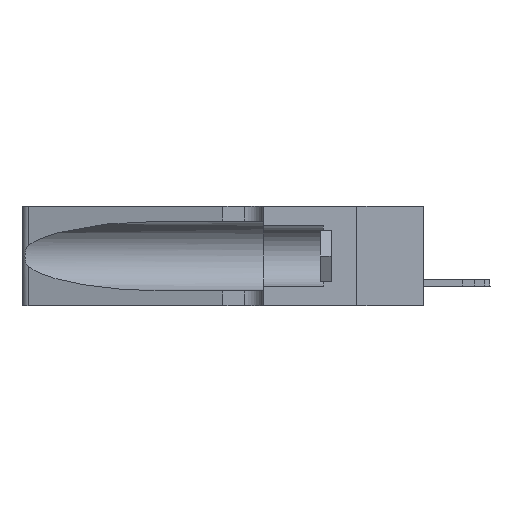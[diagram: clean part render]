
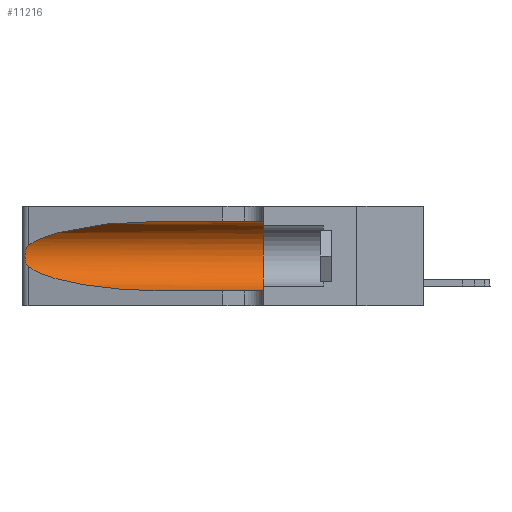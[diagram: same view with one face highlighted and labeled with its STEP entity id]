
A CAD part, left-side view. The second image highlights one B-rep face of the part: STEP entity #11216.
In plain terms, the highlighted cylindrical face has radius 3.308 mm (diameter 6.617 mm), a partial arc.
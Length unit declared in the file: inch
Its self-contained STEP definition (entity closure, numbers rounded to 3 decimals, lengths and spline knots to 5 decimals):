
#1610 = CYLINDRICAL_SURFACE ( 'NONE', #5016, 0.13025 ) ;
#2226 = DIRECTION ( 'NONE',  ( 0., 1., 0. ) ) ;
#2323 = DIRECTION ( 'NONE',  ( 0., 0., 1. ) ) ;
#2825 = AXIS2_PLACEMENT_3D ( 'NONE', #12289, #2226, #2323 ) ;
#3689 = ORIENTED_EDGE ( 'NONE', *, *, #10158, .T. ) ;
#3741 = ORIENTED_EDGE ( 'NONE', *, *, #10546, .T. ) ;
#3922 = CARTESIAN_POINT ( 'NONE',  ( 0.2373, 1.15595, 0.28018 ) ) ;
#4613 = CARTESIAN_POINT ( 'NONE',  ( 0.25787, 1.23484, 0.2124 ) ) ;
#5016 = AXIS2_PLACEMENT_3D ( 'NONE', #22524, #19921, #25355 ) ;
#5555 = CARTESIAN_POINT ( 'NONE',  ( 0.25487, 1.22718, 0.14631 ) ) ;
#5918 = EDGE_LOOP ( 'NONE', ( #3689, #3741, #30185, #19300, #8326, #10552 ) ) ;
#6093 = CARTESIAN_POINT ( 'NONE',  ( 0.1305, 0.72297, 0.31525 ) ) ;
#6492 = FACE_OUTER_BOUND ( 'NONE', #5918, .T. ) ;
#6548 = CARTESIAN_POINT ( 'NONE',  ( 0.25854, 1.2359, 0.20912 ) ) ;
#7087 = VERTEX_POINT ( 'NONE', #22837 ) ;
#8326 = ORIENTED_EDGE ( 'NONE', *, *, #11116, .F. ) ;
#10082 = EDGE_CURVE ( 'NONE', #29341, #12091, #17944, .T. ) ;
#10158 = EDGE_CURVE ( 'NONE', #7087, #11422, #27082, .T. ) ;
#10546 = EDGE_CURVE ( 'NONE', #11422, #26345, #19596, .T. ) ;
#10552 = ORIENTED_EDGE ( 'NONE', *, *, #15546, .F. ) ;
#11116 = EDGE_CURVE ( 'NONE', #26934, #12091, #32893, .T. ) ;
#11216 = ADVANCED_FACE ( 'NONE', ( #6492 ), #1610, .F. ) ;
#11422 = VERTEX_POINT ( 'NONE', #19152 ) ;
#11492 = EDGE_CURVE ( 'NONE', #26345, #29341, #21054, .T. ) ;
#11912 = CARTESIAN_POINT ( 'NONE',  ( 0.18966, 0.96281, 0.05475 ) ) ;
#12091 = VERTEX_POINT ( 'NONE', #33047 ) ;
#12289 = CARTESIAN_POINT ( 'NONE',  ( 0.1305, 0.35, 0.185 ) ) ;
#12537 = CARTESIAN_POINT ( 'NONE',  ( 0.25639, 1.23184, 0.21858 ) ) ;
#14253 = CARTESIAN_POINT ( 'NONE',  ( 0.26017, 1.23833, 0.17102 ) ) ;
#15066 = CARTESIAN_POINT ( 'NONE',  ( 0.26018, 1.23835, 0.19895 ) ) ;
#15074 = DIRECTION ( 'NONE',  ( 0., -1., 0. ) ) ;
#15171 = CARTESIAN_POINT ( 'NONE',  ( 0.26075, 1.23896, 0.19203 ) ) ;
#15546 = EDGE_CURVE ( 'NONE', #7087, #26934, #32357, .T. ) ;
#15655 = CARTESIAN_POINT ( 'NONE',  ( 0.1305, 1.61858, 0.05475 ) ) ;
#15892 = CARTESIAN_POINT ( 'NONE',  ( 0.25487, 1.22718, 0.22369 ) ) ;
#16989 = CARTESIAN_POINT ( 'NONE',  ( 0.25555, 1.22993, 0.14849 ) ) ;
#17554 = CARTESIAN_POINT ( 'NONE',  ( 0.26075, 1.23896, 0.178 ) ) ;
#17704 = DIRECTION ( 'NONE',  ( 0., -1., 0. ) ) ;
#17782 = CARTESIAN_POINT ( 'NONE',  ( 0.25856, 1.23593, 0.16098 ) ) ;
#17944 = LINE ( 'NONE', #15655, #26876 ) ;
#19152 = CARTESIAN_POINT ( 'NONE',  ( 0.25487, 1.22718, 0.22369 ) ) ;
#19300 = ORIENTED_EDGE ( 'NONE', *, *, #10082, .T. ) ;
#19596 = B_SPLINE_CURVE_WITH_KNOTS ( 'NONE', 3,
 ( #30753, #22120, #12537, #4613, #6548, #15066, #15171, #17554, #14253, #17782, #33368, #24604, #16989, #33141 ),
 .UNSPECIFIED., .F., .F.,
 ( 4, 2, 2, 2, 2, 2, 4 ),
 ( 0., 0.00027, 0.00053, 0.00107, 0.0016, 0.00187, 0.00214 ),
 .UNSPECIFIED. ) ;
#19680 = CARTESIAN_POINT ( 'NONE',  ( 0.2373, 1.15595, 0.08982 ) ) ;
#19921 = DIRECTION ( 'NONE',  ( 0., -1., 0. ) ) ;
#20162 = VECTOR ( 'NONE', #15074, 39.37008 ) ;
#21054 =( BOUNDED_CURVE ( )  B_SPLINE_CURVE ( 3, ( #32737, #19680, #11912, #27170 ),
 .UNSPECIFIED., .F., .F. ) 
 B_SPLINE_CURVE_WITH_KNOTS ( ( 4, 4 ),
 ( 3.44316, 4.71239 ),
 .UNSPECIFIED. ) 
 CURVE ( )  GEOMETRIC_REPRESENTATION_ITEM ( )  RATIONAL_B_SPLINE_CURVE ( ( 1., 0.87, 0.87, 1. ) ) 
 REPRESENTATION_ITEM ( '' )  );
#22120 = CARTESIAN_POINT ( 'NONE',  ( 0.25555, 1.22994, 0.2215 ) ) ;
#22524 = CARTESIAN_POINT ( 'NONE',  ( 0.1305, 1.61858, 0.185 ) ) ;
#22837 = CARTESIAN_POINT ( 'NONE',  ( 0.1305, 0.72297, 0.31525 ) ) ;
#24141 = CARTESIAN_POINT ( 'NONE',  ( 0.1305, 0.72297, 0.05475 ) ) ;
#24604 = CARTESIAN_POINT ( 'NONE',  ( 0.25639, 1.23186, 0.15144 ) ) ;
#25355 = DIRECTION ( 'NONE',  ( 0., 0., -1. ) ) ;
#26345 = VERTEX_POINT ( 'NONE', #5555 ) ;
#26876 = VECTOR ( 'NONE', #17704, 39.37008 ) ;
#26934 = VERTEX_POINT ( 'NONE', #29151 ) ;
#27082 =( BOUNDED_CURVE ( )  B_SPLINE_CURVE ( 3, ( #6093, #32661, #3922, #15892 ),
 .UNSPECIFIED., .F., .F. ) 
 B_SPLINE_CURVE_WITH_KNOTS ( ( 4, 4 ),
 ( 1.5708, 2.84003 ),
 .UNSPECIFIED. ) 
 CURVE ( )  GEOMETRIC_REPRESENTATION_ITEM ( )  RATIONAL_B_SPLINE_CURVE ( ( 1., 0.87, 0.87, 1. ) ) 
 REPRESENTATION_ITEM ( '' )  );
#27170 = CARTESIAN_POINT ( 'NONE',  ( 0.1305, 0.72297, 0.05475 ) ) ;
#29151 = CARTESIAN_POINT ( 'NONE',  ( 0.1305, 0.35, 0.31525 ) ) ;
#29341 = VERTEX_POINT ( 'NONE', #24141 ) ;
#30185 = ORIENTED_EDGE ( 'NONE', *, *, #11492, .T. ) ;
#30419 = CARTESIAN_POINT ( 'NONE',  ( 0.1305, 1.61858, 0.31525 ) ) ;
#30753 = CARTESIAN_POINT ( 'NONE',  ( 0.25487, 1.22718, 0.22369 ) ) ;
#32357 = LINE ( 'NONE', #30419, #20162 ) ;
#32661 = CARTESIAN_POINT ( 'NONE',  ( 0.18966, 0.96281, 0.31525 ) ) ;
#32737 = CARTESIAN_POINT ( 'NONE',  ( 0.25487, 1.22718, 0.14631 ) ) ;
#32893 = CIRCLE ( 'NONE', #2825, 0.13025 ) ;
#33047 = CARTESIAN_POINT ( 'NONE',  ( 0.1305, 0.35, 0.05475 ) ) ;
#33141 = CARTESIAN_POINT ( 'NONE',  ( 0.25487, 1.22718, 0.14631 ) ) ;
#33368 = CARTESIAN_POINT ( 'NONE',  ( 0.25789, 1.23486, 0.15765 ) ) ;
